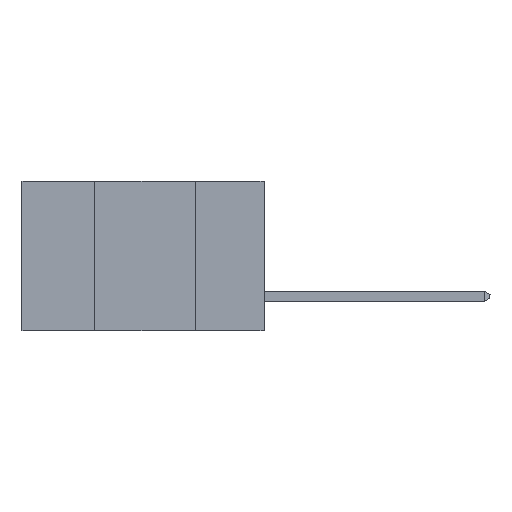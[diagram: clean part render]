
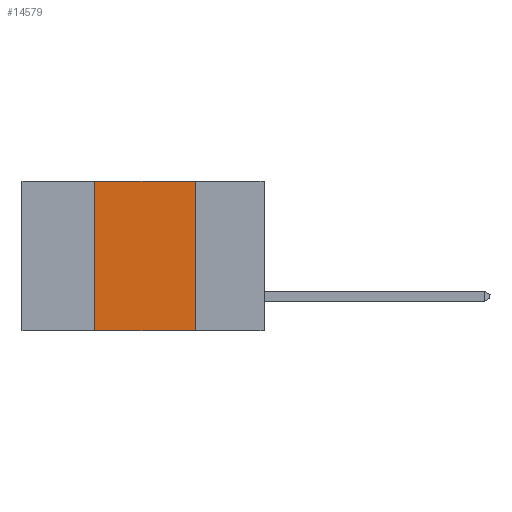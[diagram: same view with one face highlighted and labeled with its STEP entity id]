
A CAD part, left-side view. The second image highlights one B-rep face of the part: STEP entity #14579.
In plain terms, the highlighted planar face has unit normal (-1, 0, 0).
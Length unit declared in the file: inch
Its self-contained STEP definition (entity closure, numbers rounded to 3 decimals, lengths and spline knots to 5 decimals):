
#329 = CARTESIAN_POINT ( 'NONE',  ( 0., 0.42, 0. ) ) ;
#950 = EDGE_CURVE ( 'NONE', #3337, #23817, #9090, .T. ) ;
#2890 = LINE ( 'NONE', #6625, #14773 ) ;
#3337 = VERTEX_POINT ( 'NONE', #11906 ) ;
#4938 = VECTOR ( 'NONE', #12193, 39.37008 ) ;
#5701 = CARTESIAN_POINT ( 'NONE',  ( 0., 0.17, 0. ) ) ;
#6591 = ORIENTED_EDGE ( 'NONE', *, *, #950, .F. ) ;
#6625 = CARTESIAN_POINT ( 'NONE',  ( 0., 0.17, 0. ) ) ;
#8988 = EDGE_LOOP ( 'NONE', ( #20076, #6591, #12585, #24817 ) ) ;
#9090 = LINE ( 'NONE', #14469, #12112 ) ;
#10707 = EDGE_CURVE ( 'NONE', #16747, #3337, #21387, .T. ) ;
#10722 = LINE ( 'NONE', #17676, #4938 ) ;
#10865 = CARTESIAN_POINT ( 'NONE',  ( 0., 0.6, 0. ) ) ;
#11906 = CARTESIAN_POINT ( 'NONE',  ( 0., 0.42, 0. ) ) ;
#12112 = VECTOR ( 'NONE', #14552, 39.37008 ) ;
#12193 = DIRECTION ( 'NONE',  ( 0., -1., 0. ) ) ;
#12585 = ORIENTED_EDGE ( 'NONE', *, *, #10707, .F. ) ;
#12902 = DIRECTION ( 'NONE',  ( 0., 0., -1. ) ) ;
#14469 = CARTESIAN_POINT ( 'NONE',  ( 0., 0.6, 0. ) ) ;
#14552 = DIRECTION ( 'NONE',  ( 0., -1., 0. ) ) ;
#14579 = ADVANCED_FACE ( 'NONE', ( #21461 ), #16657, .F. ) ;
#14773 = VECTOR ( 'NONE', #16403, 39.37008 ) ;
#16403 = DIRECTION ( 'NONE',  ( 0., 0., -1. ) ) ;
#16657 = PLANE ( 'NONE',  #24294 ) ;
#16747 = VERTEX_POINT ( 'NONE', #21321 ) ;
#16780 = VECTOR ( 'NONE', #17889, 39.37008 ) ;
#17676 = CARTESIAN_POINT ( 'NONE',  ( 0., 0.6, -0.37 ) ) ;
#17710 = EDGE_CURVE ( 'NONE', #23817, #22935, #2890, .T. ) ;
#17889 = DIRECTION ( 'NONE',  ( 0., 0., 1. ) ) ;
#18688 = DIRECTION ( 'NONE',  ( 1., 0., 0. ) ) ;
#19776 = EDGE_CURVE ( 'NONE', #16747, #22935, #10722, .T. ) ;
#20076 = ORIENTED_EDGE ( 'NONE', *, *, #17710, .F. ) ;
#21321 = CARTESIAN_POINT ( 'NONE',  ( 0., 0.42, -0.37 ) ) ;
#21387 = LINE ( 'NONE', #329, #16780 ) ;
#21461 = FACE_OUTER_BOUND ( 'NONE', #8988, .T. ) ;
#22935 = VERTEX_POINT ( 'NONE', #24736 ) ;
#23817 = VERTEX_POINT ( 'NONE', #5701 ) ;
#24294 = AXIS2_PLACEMENT_3D ( 'NONE', #10865, #18688, #12902 ) ;
#24736 = CARTESIAN_POINT ( 'NONE',  ( 0., 0.17, -0.37 ) ) ;
#24817 = ORIENTED_EDGE ( 'NONE', *, *, #19776, .T. ) ;
